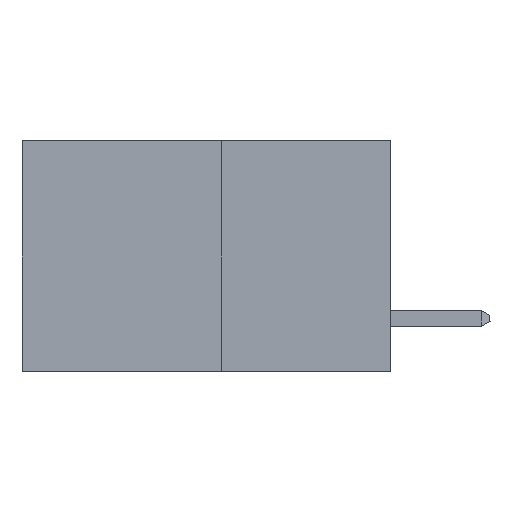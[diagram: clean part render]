
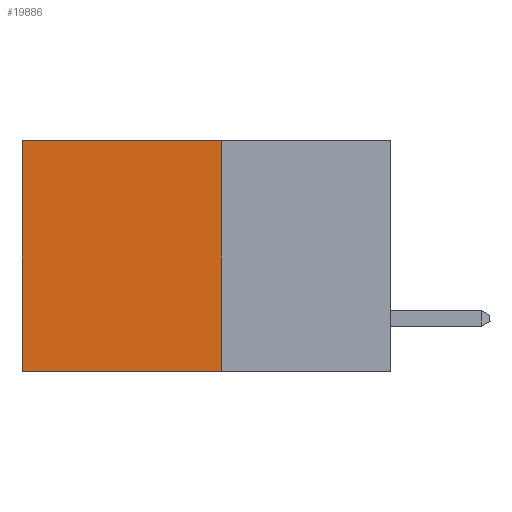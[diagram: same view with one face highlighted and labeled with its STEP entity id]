
A CAD part, left-side view. The second image highlights one B-rep face of the part: STEP entity #19886.
In plain terms, the highlighted planar face has unit normal (-1, 0, 0).
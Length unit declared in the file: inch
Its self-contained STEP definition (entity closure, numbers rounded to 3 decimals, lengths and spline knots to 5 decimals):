
#98 = CARTESIAN_POINT ( 'NONE',  ( 0.277, 0.27, -0.37 ) ) ;
#1950 = CARTESIAN_POINT ( 'NONE',  ( 0.277, 0.27, -0.37 ) ) ;
#2978 = LINE ( 'NONE', #1950, #19076 ) ;
#3994 = EDGE_CURVE ( 'NONE', #17931, #14182, #5808, .T. ) ;
#4724 = CARTESIAN_POINT ( 'NONE',  ( 0.277, 0.59, -0.37 ) ) ;
#5740 = DIRECTION ( 'NONE',  ( 0., 0., -1. ) ) ;
#5808 = LINE ( 'NONE', #9732, #13630 ) ;
#6144 = VECTOR ( 'NONE', #11682, 39.37008 ) ;
#6262 = ORIENTED_EDGE ( 'NONE', *, *, #3994, .T. ) ;
#7781 = VECTOR ( 'NONE', #15061, 39.37008 ) ;
#8540 = VERTEX_POINT ( 'NONE', #10142 ) ;
#9415 = DIRECTION ( 'NONE',  ( 0., 0., -1. ) ) ;
#9732 = CARTESIAN_POINT ( 'NONE',  ( 0.277, 0.59, -0.37 ) ) ;
#10096 = CARTESIAN_POINT ( 'NONE',  ( 0.277, 0.27, 0. ) ) ;
#10142 = CARTESIAN_POINT ( 'NONE',  ( 0.277, 0.27, 0. ) ) ;
#10456 = ORIENTED_EDGE ( 'NONE', *, *, #15009, .F. ) ;
#11239 = AXIS2_PLACEMENT_3D ( 'NONE', #13532, #18045, #5740 ) ;
#11682 = DIRECTION ( 'NONE',  ( 0., 1., 0. ) ) ;
#13039 = CARTESIAN_POINT ( 'NONE',  ( 0.277, 0.59, 0. ) ) ;
#13230 = EDGE_CURVE ( 'NONE', #8540, #17931, #14907, .T. ) ;
#13523 = CARTESIAN_POINT ( 'NONE',  ( 0.277, 0.27, -0.37 ) ) ;
#13532 = CARTESIAN_POINT ( 'NONE',  ( 0.277, 0.27, -0.37 ) ) ;
#13630 = VECTOR ( 'NONE', #9415, 39.37008 ) ;
#13775 = EDGE_LOOP ( 'NONE', ( #6262, #10456, #14549, #15031 ) ) ;
#14182 = VERTEX_POINT ( 'NONE', #4724 ) ;
#14541 = DIRECTION ( 'NONE',  ( 0., 1., 0. ) ) ;
#14549 = ORIENTED_EDGE ( 'NONE', *, *, #19363, .F. ) ;
#14907 = LINE ( 'NONE', #10096, #6144 ) ;
#15009 = EDGE_CURVE ( 'NONE', #20241, #14182, #2978, .T. ) ;
#15031 = ORIENTED_EDGE ( 'NONE', *, *, #13230, .T. ) ;
#15061 = DIRECTION ( 'NONE',  ( 0., 0., -1. ) ) ;
#15072 = PLANE ( 'NONE',  #11239 ) ;
#15995 = LINE ( 'NONE', #13523, #7781 ) ;
#17904 = FACE_OUTER_BOUND ( 'NONE', #13775, .T. ) ;
#17931 = VERTEX_POINT ( 'NONE', #13039 ) ;
#18045 = DIRECTION ( 'NONE',  ( 1., 0., 0. ) ) ;
#19076 = VECTOR ( 'NONE', #14541, 39.37008 ) ;
#19363 = EDGE_CURVE ( 'NONE', #8540, #20241, #15995, .T. ) ;
#19886 = ADVANCED_FACE ( 'NONE', ( #17904 ), #15072, .F. ) ;
#20241 = VERTEX_POINT ( 'NONE', #98 ) ;
